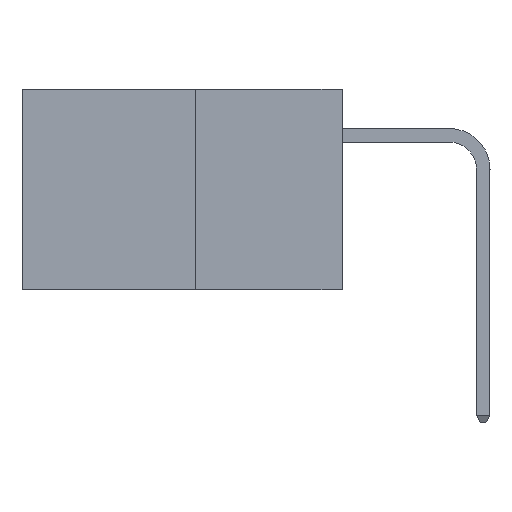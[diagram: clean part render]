
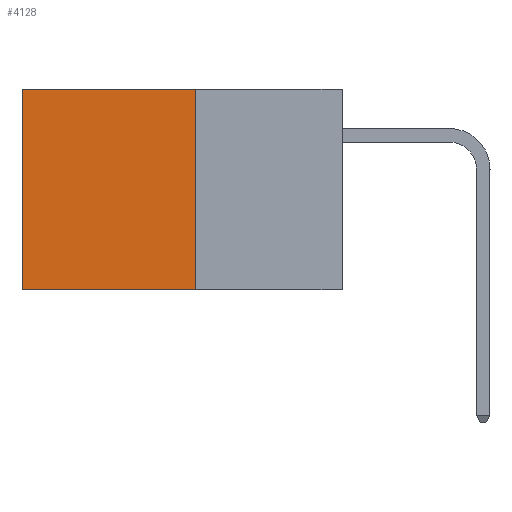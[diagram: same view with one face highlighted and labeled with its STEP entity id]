
A CAD part, left-side view. The second image highlights one B-rep face of the part: STEP entity #4128.
In plain terms, the highlighted planar face has unit normal (-1, 0, 0).
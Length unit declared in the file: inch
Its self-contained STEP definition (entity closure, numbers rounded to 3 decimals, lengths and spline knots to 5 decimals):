
#1355 = ORIENTED_EDGE ( 'NONE', *, *, #13497, .T. ) ;
#1640 = EDGE_LOOP ( 'NONE', ( #1355, #4781, #14927, #17453 ) ) ;
#1679 = CARTESIAN_POINT ( 'NONE',  ( 0.277, 0.59, -0.37 ) ) ;
#2482 = VERTEX_POINT ( 'NONE', #2819 ) ;
#2819 = CARTESIAN_POINT ( 'NONE',  ( 0.277, 0.27, 0. ) ) ;
#2908 = VECTOR ( 'NONE', #5174, 39.37008 ) ;
#3670 = CARTESIAN_POINT ( 'NONE',  ( 0.277, 0.59, 0. ) ) ;
#4128 = ADVANCED_FACE ( 'NONE', ( #18921 ), #17925, .F. ) ;
#4781 = ORIENTED_EDGE ( 'NONE', *, *, #6521, .F. ) ;
#4881 = EDGE_CURVE ( 'NONE', #2482, #13680, #5675, .T. ) ;
#5145 = VECTOR ( 'NONE', #11380, 39.37008 ) ;
#5174 = DIRECTION ( 'NONE',  ( 0., 1., 0. ) ) ;
#5675 = LINE ( 'NONE', #13897, #5145 ) ;
#6422 = AXIS2_PLACEMENT_3D ( 'NONE', #17931, #17626, #17569 ) ;
#6521 = EDGE_CURVE ( 'NONE', #13680, #12397, #20346, .T. ) ;
#6843 = DIRECTION ( 'NONE',  ( 0., 0., -1. ) ) ;
#8051 = VECTOR ( 'NONE', #6843, 39.37008 ) ;
#8522 = CARTESIAN_POINT ( 'NONE',  ( 0.277, 0.27, 0. ) ) ;
#11380 = DIRECTION ( 'NONE',  ( 0., 0., -1. ) ) ;
#11481 = EDGE_CURVE ( 'NONE', #2482, #16578, #16493, .T. ) ;
#12397 = VERTEX_POINT ( 'NONE', #12568 ) ;
#12568 = CARTESIAN_POINT ( 'NONE',  ( 0.277, 0.59, -0.37 ) ) ;
#12578 = LINE ( 'NONE', #1679, #8051 ) ;
#13495 = CARTESIAN_POINT ( 'NONE',  ( 0.277, 0.27, -0.37 ) ) ;
#13497 = EDGE_CURVE ( 'NONE', #16578, #12397, #12578, .T. ) ;
#13640 = DIRECTION ( 'NONE',  ( 0., 1., 0. ) ) ;
#13680 = VERTEX_POINT ( 'NONE', #14162 ) ;
#13897 = CARTESIAN_POINT ( 'NONE',  ( 0.277, 0.27, -0.37 ) ) ;
#14162 = CARTESIAN_POINT ( 'NONE',  ( 0.277, 0.27, -0.37 ) ) ;
#14612 = VECTOR ( 'NONE', #13640, 39.37008 ) ;
#14927 = ORIENTED_EDGE ( 'NONE', *, *, #4881, .F. ) ;
#16493 = LINE ( 'NONE', #8522, #2908 ) ;
#16578 = VERTEX_POINT ( 'NONE', #3670 ) ;
#17453 = ORIENTED_EDGE ( 'NONE', *, *, #11481, .T. ) ;
#17569 = DIRECTION ( 'NONE',  ( 0., 0., -1. ) ) ;
#17626 = DIRECTION ( 'NONE',  ( 1., 0., 0. ) ) ;
#17925 = PLANE ( 'NONE',  #6422 ) ;
#17931 = CARTESIAN_POINT ( 'NONE',  ( 0.277, 0.27, -0.37 ) ) ;
#18921 = FACE_OUTER_BOUND ( 'NONE', #1640, .T. ) ;
#20346 = LINE ( 'NONE', #13495, #14612 ) ;
